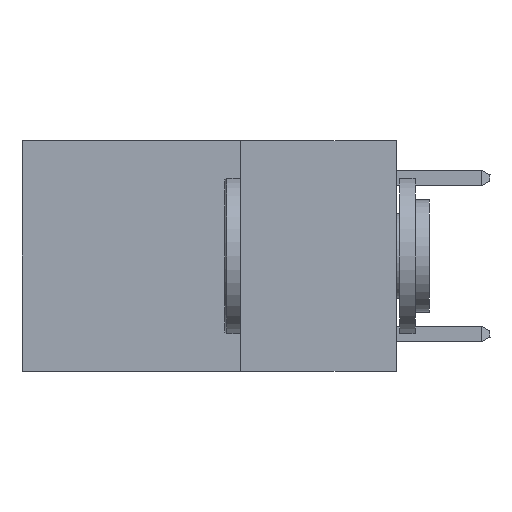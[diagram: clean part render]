
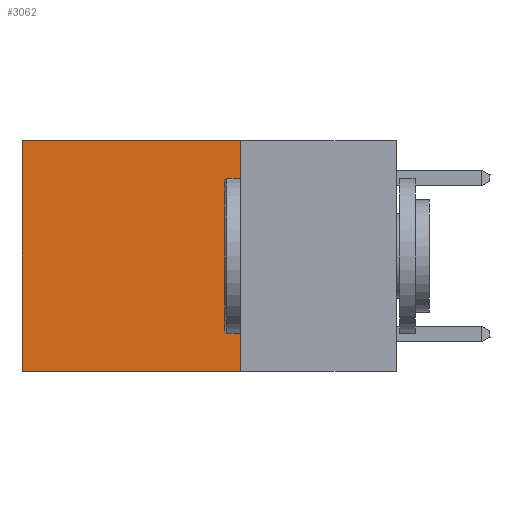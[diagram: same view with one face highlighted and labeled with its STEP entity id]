
A CAD part, left-side view. The second image highlights one B-rep face of the part: STEP entity #3062.
In plain terms, the highlighted planar face has unit normal (-1, 0, 0).
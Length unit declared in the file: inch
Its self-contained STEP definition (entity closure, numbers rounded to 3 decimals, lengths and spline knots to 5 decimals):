
#427 = DIRECTION ( 'NONE',  ( 0., 0., -1. ) ) ;
#914 = LINE ( 'NONE', #10835, #31921 ) ;
#1712 = EDGE_CURVE ( 'NONE', #19056, #30781, #914, .T. ) ;
#3062 = ADVANCED_FACE ( 'NONE', ( #4362 ), #6625, .F. ) ;
#3250 = EDGE_CURVE ( 'NONE', #24829, #30781, #8066, .T. ) ;
#4362 = FACE_OUTER_BOUND ( 'NONE', #30547, .T. ) ;
#4639 = ORIENTED_EDGE ( 'NONE', *, *, #1712, .F. ) ;
#6113 = VECTOR ( 'NONE', #6517, 39.37008 ) ;
#6517 = DIRECTION ( 'NONE',  ( 0., 0., -1. ) ) ;
#6625 = PLANE ( 'NONE',  #16338 ) ;
#6671 = CARTESIAN_POINT ( 'NONE',  ( 0.2625, 0.25, 0. ) ) ;
#8066 = LINE ( 'NONE', #17679, #30946 ) ;
#8201 = DIRECTION ( 'NONE',  ( 0., 1., 0. ) ) ;
#8678 = CARTESIAN_POINT ( 'NONE',  ( 0.2625, 0.6, 0. ) ) ;
#9209 = CARTESIAN_POINT ( 'NONE',  ( 0.2625, 0.25, 0. ) ) ;
#9372 = DIRECTION ( 'NONE',  ( 1., 0., 0. ) ) ;
#10196 = EDGE_CURVE ( 'NONE', #16666, #24829, #23355, .T. ) ;
#10835 = CARTESIAN_POINT ( 'NONE',  ( 0.2625, 0.25, -0.37 ) ) ;
#15699 = ORIENTED_EDGE ( 'NONE', *, *, #3250, .T. ) ;
#15703 = CARTESIAN_POINT ( 'NONE',  ( 0.2625, 0.6, -0.37 ) ) ;
#16148 = VECTOR ( 'NONE', #8201, 39.37008 ) ;
#16315 = EDGE_CURVE ( 'NONE', #16666, #19056, #28845, .T. ) ;
#16338 = AXIS2_PLACEMENT_3D ( 'NONE', #9209, #9372, #16712 ) ;
#16666 = VERTEX_POINT ( 'NONE', #29282 ) ;
#16712 = DIRECTION ( 'NONE',  ( 0., 0., -1. ) ) ;
#17679 = CARTESIAN_POINT ( 'NONE',  ( 0.2625, 0.6, 0. ) ) ;
#18108 = ORIENTED_EDGE ( 'NONE', *, *, #16315, .F. ) ;
#19056 = VERTEX_POINT ( 'NONE', #26434 ) ;
#22886 = CARTESIAN_POINT ( 'NONE',  ( 0.2625, 0.25, 0. ) ) ;
#23355 = LINE ( 'NONE', #22886, #16148 ) ;
#23380 = ORIENTED_EDGE ( 'NONE', *, *, #10196, .T. ) ;
#24829 = VERTEX_POINT ( 'NONE', #8678 ) ;
#26434 = CARTESIAN_POINT ( 'NONE',  ( 0.2625, 0.25, -0.37 ) ) ;
#27952 = DIRECTION ( 'NONE',  ( 0., 1., 0. ) ) ;
#28845 = LINE ( 'NONE', #6671, #6113 ) ;
#29282 = CARTESIAN_POINT ( 'NONE',  ( 0.2625, 0.25, 0. ) ) ;
#30547 = EDGE_LOOP ( 'NONE', ( #15699, #4639, #18108, #23380 ) ) ;
#30781 = VERTEX_POINT ( 'NONE', #15703 ) ;
#30946 = VECTOR ( 'NONE', #427, 39.37008 ) ;
#31921 = VECTOR ( 'NONE', #27952, 39.37008 ) ;
